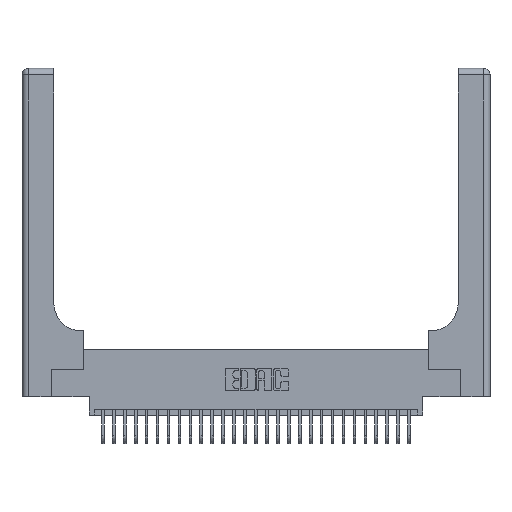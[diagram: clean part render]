
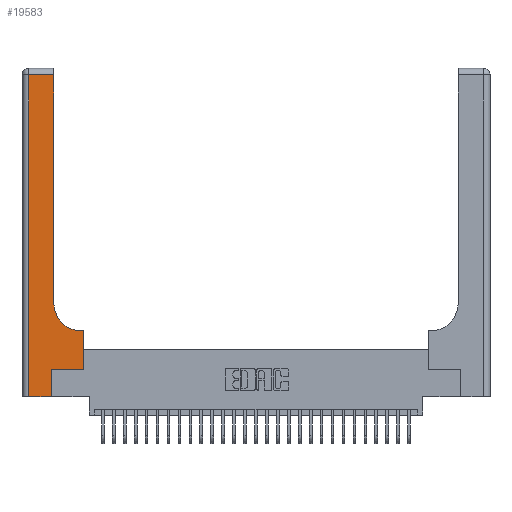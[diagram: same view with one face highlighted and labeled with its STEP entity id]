
A CAD part, top view. The second image highlights one B-rep face of the part: STEP entity #19583.
In plain terms, the highlighted planar face has unit normal (0, 0, 1).
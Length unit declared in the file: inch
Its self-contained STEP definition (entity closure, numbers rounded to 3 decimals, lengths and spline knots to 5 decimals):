
#763 = DIRECTION ( 'NONE',  ( -1., 0., 0. ) ) ;
#1230 = DIRECTION ( 'NONE',  ( 0., 1., 0. ) ) ;
#1467 = ORIENTED_EDGE ( 'NONE', *, *, #14130, .T. ) ;
#1763 = DIRECTION ( 'NONE',  ( 1., 0., 0. ) ) ;
#1862 = VERTEX_POINT ( 'NONE', #11723 ) ;
#2911 = CARTESIAN_POINT ( 'NONE',  ( 0.2915, 2.94, 0.37 ) ) ;
#3304 = VECTOR ( 'NONE', #1763, 39.37008 ) ;
#3540 = CARTESIAN_POINT ( 'NONE',  ( 0.269, 0., 0.37 ) ) ;
#3604 = CARTESIAN_POINT ( 'NONE',  ( 0.2915, 3., 0.37 ) ) ;
#3836 = CARTESIAN_POINT ( 'NONE',  ( 0., 0., 0.37 ) ) ;
#4297 = ORIENTED_EDGE ( 'NONE', *, *, #10851, .T. ) ;
#5022 = LINE ( 'NONE', #14142, #22100 ) ;
#5561 = CARTESIAN_POINT ( 'NONE',  ( 0.5585, 0.25, 0.37 ) ) ;
#5851 = LINE ( 'NONE', #26418, #16965 ) ;
#5867 = DIRECTION ( 'NONE',  ( 0., 1., 0. ) ) ;
#5995 = DIRECTION ( 'NONE',  ( 1., 0., 0. ) ) ;
#6072 = ORIENTED_EDGE ( 'NONE', *, *, #15944, .T. ) ;
#6257 = CARTESIAN_POINT ( 'NONE',  ( 0.2915, 0.6, 0.37 ) ) ;
#6839 = LINE ( 'NONE', #6257, #17973 ) ;
#6945 = VERTEX_POINT ( 'NONE', #11579 ) ;
#7388 = EDGE_CURVE ( 'NONE', #21422, #26661, #5851, .T. ) ;
#8377 = CARTESIAN_POINT ( 'NONE',  ( 0.5415, 0.85, 0.37 ) ) ;
#9321 = DIRECTION ( 'NONE',  ( -1., 0., 0. ) ) ;
#9772 = AXIS2_PLACEMENT_3D ( 'NONE', #22599, #22701, #9321 ) ;
#10603 = DIRECTION ( 'NONE',  ( 1., 0., 0. ) ) ;
#10851 = EDGE_CURVE ( 'NONE', #15679, #6945, #5022, .T. ) ;
#11047 = CIRCLE ( 'NONE', #15614, 0.25 ) ;
#11579 = CARTESIAN_POINT ( 'NONE',  ( 0.06, 2.94, 0.37 ) ) ;
#11723 = CARTESIAN_POINT ( 'NONE',  ( 0.269, 0., 0.37 ) ) ;
#11725 = CARTESIAN_POINT ( 'NONE',  ( 0.269, 0.25, 0.37 ) ) ;
#12268 = ORIENTED_EDGE ( 'NONE', *, *, #23569, .T. ) ;
#14130 = EDGE_CURVE ( 'NONE', #23352, #24190, #11047, .T. ) ;
#14142 = CARTESIAN_POINT ( 'NONE',  ( 0., 2.94, 0.37 ) ) ;
#14284 = DIRECTION ( 'NONE',  ( 0., -1., 0. ) ) ;
#14845 = VECTOR ( 'NONE', #5995, 39.37008 ) ;
#15061 = ORIENTED_EDGE ( 'NONE', *, *, #26553, .T. ) ;
#15287 = EDGE_CURVE ( 'NONE', #1862, #18262, #24343, .T. ) ;
#15356 = EDGE_CURVE ( 'NONE', #16847, #1862, #20106, .T. ) ;
#15385 = ORIENTED_EDGE ( 'NONE', *, *, #22416, .T. ) ;
#15614 = AXIS2_PLACEMENT_3D ( 'NONE', #8377, #23997, #10603 ) ;
#15679 = VERTEX_POINT ( 'NONE', #2911 ) ;
#15746 = ORIENTED_EDGE ( 'NONE', *, *, #7388, .T. ) ;
#15944 = EDGE_CURVE ( 'NONE', #26661, #23352, #6839, .T. ) ;
#16243 = VECTOR ( 'NONE', #1230, 39.37008 ) ;
#16847 = VERTEX_POINT ( 'NONE', #18344 ) ;
#16965 = VECTOR ( 'NONE', #28639, 39.37008 ) ;
#17083 = LINE ( 'NONE', #25465, #23020 ) ;
#17973 = VECTOR ( 'NONE', #19574, 39.37008 ) ;
#18034 = CARTESIAN_POINT ( 'NONE',  ( 0.5415, 0.6, 0.37 ) ) ;
#18190 = PLANE ( 'NONE',  #9772 ) ;
#18262 = VERTEX_POINT ( 'NONE', #11725 ) ;
#18344 = CARTESIAN_POINT ( 'NONE',  ( 0.06, 0., 0.37 ) ) ;
#18922 = ORIENTED_EDGE ( 'NONE', *, *, #15356, .T. ) ;
#19574 = DIRECTION ( 'NONE',  ( -1., 0., 0. ) ) ;
#19583 = ADVANCED_FACE ( 'NONE', ( #20042 ), #18190, .F. ) ;
#19898 = CARTESIAN_POINT ( 'NONE',  ( 0.5585, 0.6, 0.37 ) ) ;
#20042 = FACE_OUTER_BOUND ( 'NONE', #28570, .T. ) ;
#20106 = LINE ( 'NONE', #3836, #14845 ) ;
#21422 = VERTEX_POINT ( 'NONE', #5561 ) ;
#22100 = VECTOR ( 'NONE', #763, 39.37008 ) ;
#22398 = LINE ( 'NONE', #3604, #27604 ) ;
#22416 = EDGE_CURVE ( 'NONE', #24190, #15679, #22398, .T. ) ;
#22599 = CARTESIAN_POINT ( 'NONE',  ( 0., 3., 0.37 ) ) ;
#22701 = DIRECTION ( 'NONE',  ( 0., 0., -1. ) ) ;
#23020 = VECTOR ( 'NONE', #14284, 39.37008 ) ;
#23352 = VERTEX_POINT ( 'NONE', #18034 ) ;
#23569 = EDGE_CURVE ( 'NONE', #6945, #16847, #17083, .T. ) ;
#23997 = DIRECTION ( 'NONE',  ( 0., 0., -1. ) ) ;
#24190 = VERTEX_POINT ( 'NONE', #25226 ) ;
#24343 = LINE ( 'NONE', #3540, #16243 ) ;
#25226 = CARTESIAN_POINT ( 'NONE',  ( 0.2915, 0.85, 0.37 ) ) ;
#25465 = CARTESIAN_POINT ( 'NONE',  ( 0.06, 3., 0.37 ) ) ;
#26260 = ORIENTED_EDGE ( 'NONE', *, *, #15287, .T. ) ;
#26418 = CARTESIAN_POINT ( 'NONE',  ( 0.5585, 0.25, 0.37 ) ) ;
#26553 = EDGE_CURVE ( 'NONE', #18262, #21422, #27699, .T. ) ;
#26661 = VERTEX_POINT ( 'NONE', #19898 ) ;
#27604 = VECTOR ( 'NONE', #5867, 39.37008 ) ;
#27699 = LINE ( 'NONE', #28383, #3304 ) ;
#28383 = CARTESIAN_POINT ( 'NONE',  ( 0.269, 0.25, 0.37 ) ) ;
#28570 = EDGE_LOOP ( 'NONE', ( #15385, #4297, #12268, #18922, #26260, #15061, #15746, #6072, #1467 ) ) ;
#28639 = DIRECTION ( 'NONE',  ( 0., 1., 0. ) ) ;
